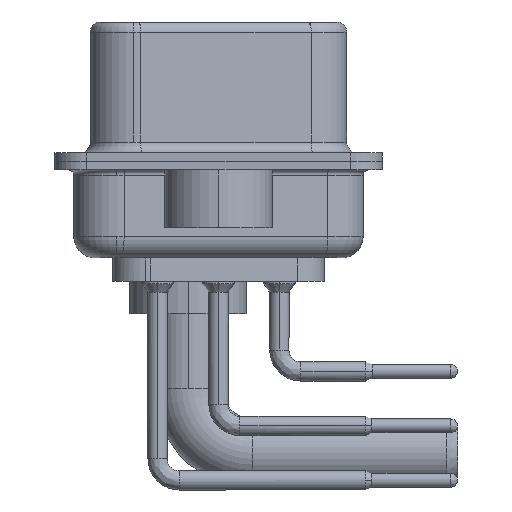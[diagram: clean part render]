
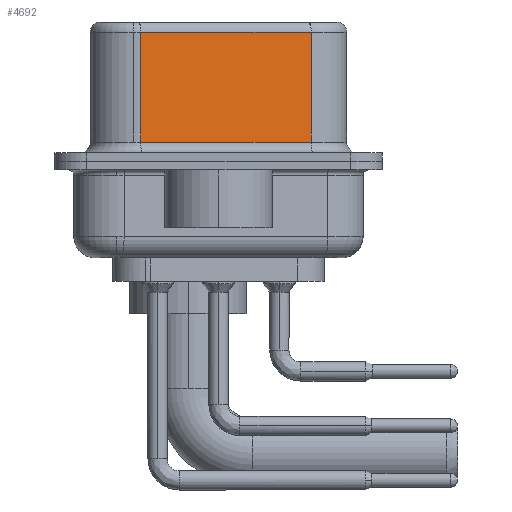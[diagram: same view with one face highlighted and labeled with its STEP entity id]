
A CAD part, left-side view. The second image highlights one B-rep face of the part: STEP entity #4692.
In plain terms, the highlighted planar face has unit normal (-0.985, -0.174, 0).
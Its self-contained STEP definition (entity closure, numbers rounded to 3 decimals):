
#142 = CARTESIAN_POINT ( 'NONE',  ( 3.73, 3.628, 6.02 ) ) ;
#2951 = PLANE ( 'NONE',  #5541 ) ;
#3255 = CARTESIAN_POINT ( 'NONE',  ( 3.73, 3.628, 0.9 ) ) ;
#3905 = LINE ( 'NONE', #4271, #31991 ) ;
#4271 = CARTESIAN_POINT ( 'NONE',  ( 5.132, -4.322, 0.9 ) ) ;
#4692 = ADVANCED_FACE ( 'NONE', ( #19646 ), #2951, .F. ) ;
#5541 = AXIS2_PLACEMENT_3D ( 'NONE', #5695, #16891, #6054 ) ;
#5695 = CARTESIAN_POINT ( 'NONE',  ( 5.132, -4.322, 6.52 ) ) ;
#5852 = EDGE_CURVE ( 'NONE', #15903, #7932, #15636, .T. ) ;
#6054 = DIRECTION ( 'NONE',  ( -0.174, 0.985, 0. ) ) ;
#7398 = ORIENTED_EDGE ( 'NONE', *, *, #16370, .T. ) ;
#7932 = VERTEX_POINT ( 'NONE', #3255 ) ;
#9377 = CARTESIAN_POINT ( 'NONE',  ( 5.132, -4.322, 6.52 ) ) ;
#9495 = VECTOR ( 'NONE', #16598, 1000. ) ;
#9590 = ORIENTED_EDGE ( 'NONE', *, *, #26751, .F. ) ;
#9714 = ORIENTED_EDGE ( 'NONE', *, *, #5852, .T. ) ;
#10261 = EDGE_CURVE ( 'NONE', #7932, #21773, #3905, .T. ) ;
#13673 = LINE ( 'NONE', #30376, #9495 ) ;
#14897 = LINE ( 'NONE', #9377, #30789 ) ;
#15636 = LINE ( 'NONE', #18566, #29643 ) ;
#15903 = VERTEX_POINT ( 'NONE', #142 ) ;
#16370 = EDGE_CURVE ( 'NONE', #31868, #15903, #13673, .T. ) ;
#16598 = DIRECTION ( 'NONE',  ( -0.174, 0.985, 0. ) ) ;
#16891 = DIRECTION ( 'NONE',  ( 0.985, 0.174, 0. ) ) ;
#18566 = CARTESIAN_POINT ( 'NONE',  ( 3.73, 3.628, 6.52 ) ) ;
#19337 = CARTESIAN_POINT ( 'NONE',  ( 5.132, -4.322, 0.9 ) ) ;
#19646 = FACE_OUTER_BOUND ( 'NONE', #21672, .T. ) ;
#20949 = CARTESIAN_POINT ( 'NONE',  ( 5.132, -4.322, 6.02 ) ) ;
#21672 = EDGE_LOOP ( 'NONE', ( #9590, #7398, #9714, #24405 ) ) ;
#21773 = VERTEX_POINT ( 'NONE', #19337 ) ;
#24405 = ORIENTED_EDGE ( 'NONE', *, *, #10261, .T. ) ;
#26094 = DIRECTION ( 'NONE',  ( 0., 0., -1. ) ) ;
#26751 = EDGE_CURVE ( 'NONE', #31868, #21773, #14897, .T. ) ;
#29643 = VECTOR ( 'NONE', #29753, 1000. ) ;
#29753 = DIRECTION ( 'NONE',  ( 0., 0., -1. ) ) ;
#30376 = CARTESIAN_POINT ( 'NONE',  ( 5.132, -4.322, 6.02 ) ) ;
#30789 = VECTOR ( 'NONE', #26094, 1000. ) ;
#31868 = VERTEX_POINT ( 'NONE', #20949 ) ;
#31991 = VECTOR ( 'NONE', #34558, 1000. ) ;
#34558 = DIRECTION ( 'NONE',  ( 0.174, -0.985, 0. ) ) ;
